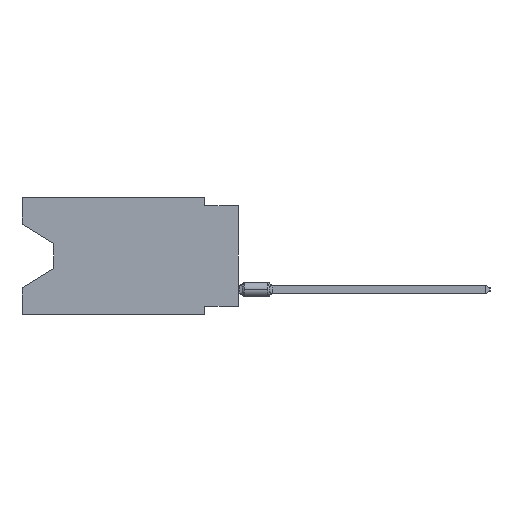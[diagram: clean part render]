
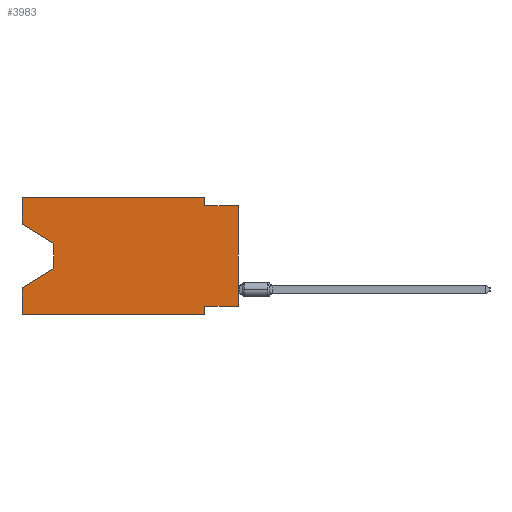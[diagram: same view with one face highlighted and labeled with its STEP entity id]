
A CAD part, left-side view. The second image highlights one B-rep face of the part: STEP entity #3983.
In plain terms, the highlighted planar face has unit normal (-1, 0, 0).
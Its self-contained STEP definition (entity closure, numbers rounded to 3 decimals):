
#249 = DIRECTION ( 'NONE',  ( 0., 0., 1. ) ) ;
#2544 = EDGE_CURVE ( 'NONE', #77701, #32352, #34237, .T. ) ;
#3983 = ADVANCED_FACE ( 'NONE', ( #42698 ), #12333, .F. ) ;
#5092 = DIRECTION ( 'NONE',  ( 0., 0., -1. ) ) ;
#7865 = VECTOR ( 'NONE', #76182, 1000. ) ;
#8477 = DIRECTION ( 'NONE',  ( 0., 1., 0. ) ) ;
#9603 = VECTOR ( 'NONE', #49959, 1000. ) ;
#9674 = CARTESIAN_POINT ( 'NONE',  ( 0., 0., -8.255 ) ) ;
#10720 = ORIENTED_EDGE ( 'NONE', *, *, #47616, .F. ) ;
#11368 = DIRECTION ( 'NONE',  ( 0., 0., 1. ) ) ;
#11590 = CARTESIAN_POINT ( 'NONE',  ( 0., 16.383, 0. ) ) ;
#12333 = PLANE ( 'NONE',  #65677 ) ;
#13125 = CARTESIAN_POINT ( 'NONE',  ( 0., 0., -0.635 ) ) ;
#13691 = VERTEX_POINT ( 'NONE', #33695 ) ;
#14118 = EDGE_LOOP ( 'NONE', ( #53825, #48049, #63645, #10720, #72800, #54632, #21055, #39411, #59504, #50692, #37069, #33156 ) ) ;
#15227 = DIRECTION ( 'NONE',  ( 0., -1., 0. ) ) ;
#15366 = VECTOR ( 'NONE', #54154, 1000. ) ;
#15761 = LINE ( 'NONE', #9674, #18253 ) ;
#17063 = VERTEX_POINT ( 'NONE', #44569 ) ;
#18253 = VECTOR ( 'NONE', #8477, 1000. ) ;
#20013 = VERTEX_POINT ( 'NONE', #76857 ) ;
#21055 = ORIENTED_EDGE ( 'NONE', *, *, #52044, .F. ) ;
#21905 = VERTEX_POINT ( 'NONE', #74834 ) ;
#25307 = LINE ( 'NONE', #79492, #9603 ) ;
#28143 = VERTEX_POINT ( 'NONE', #28400 ) ;
#28400 = CARTESIAN_POINT ( 'NONE',  ( 0., 2.54, -8.255 ) ) ;
#28641 = CARTESIAN_POINT ( 'NONE',  ( 0., 2.54, 0. ) ) ;
#30608 = LINE ( 'NONE', #11590, #71094 ) ;
#30962 = CARTESIAN_POINT ( 'NONE',  ( 0., 2.54, -0.635 ) ) ;
#31769 = CARTESIAN_POINT ( 'NONE',  ( 0., 2.54, 0. ) ) ;
#32124 = LINE ( 'NONE', #62843, #7865 ) ;
#32352 = VERTEX_POINT ( 'NONE', #72985 ) ;
#33156 = ORIENTED_EDGE ( 'NONE', *, *, #76078, .F. ) ;
#33184 = VECTOR ( 'NONE', #67475, 1000. ) ;
#33695 = CARTESIAN_POINT ( 'NONE',  ( 0., 0., -0.635 ) ) ;
#34237 = LINE ( 'NONE', #58502, #55093 ) ;
#35611 = EDGE_CURVE ( 'NONE', #21905, #17063, #32124, .T. ) ;
#36642 = LINE ( 'NONE', #31769, #58077 ) ;
#37069 = ORIENTED_EDGE ( 'NONE', *, *, #60213, .F. ) ;
#38857 = CARTESIAN_POINT ( 'NONE',  ( 0., 16.383, 0. ) ) ;
#39411 = ORIENTED_EDGE ( 'NONE', *, *, #66450, .T. ) ;
#39468 = VERTEX_POINT ( 'NONE', #38857 ) ;
#40224 = DIRECTION ( 'NONE',  ( 0., -1., 0. ) ) ;
#40738 = EDGE_CURVE ( 'NONE', #61234, #20013, #78411, .T. ) ;
#41652 = CARTESIAN_POINT ( 'NONE',  ( 0., 16.383, 0. ) ) ;
#41733 = CARTESIAN_POINT ( 'NONE',  ( 0., 0., 0. ) ) ;
#42698 = FACE_OUTER_BOUND ( 'NONE', #14118, .T. ) ;
#44569 = CARTESIAN_POINT ( 'NONE',  ( 0., 16.383, -6.852 ) ) ;
#45139 = EDGE_CURVE ( 'NONE', #20013, #21905, #25307, .T. ) ;
#46511 = VECTOR ( 'NONE', #62462, 1000. ) ;
#47616 = EDGE_CURVE ( 'NONE', #77701, #17063, #48108, .T. ) ;
#47877 = LINE ( 'NONE', #66467, #68755 ) ;
#48049 = ORIENTED_EDGE ( 'NONE', *, *, #45139, .T. ) ;
#48108 = LINE ( 'NONE', #41652, #33184 ) ;
#49320 = VERTEX_POINT ( 'NONE', #71123 ) ;
#49959 = DIRECTION ( 'NONE',  ( 0., 0., -1. ) ) ;
#50362 = EDGE_CURVE ( 'NONE', #28143, #32352, #63174, .T. ) ;
#50692 = ORIENTED_EDGE ( 'NONE', *, *, #67347, .F. ) ;
#51031 = CARTESIAN_POINT ( 'NONE',  ( 0., 2.54, -8.89 ) ) ;
#52044 = EDGE_CURVE ( 'NONE', #49320, #28143, #15761, .T. ) ;
#53682 = CARTESIAN_POINT ( 'NONE',  ( 0., 16.383, -8.89 ) ) ;
#53825 = ORIENTED_EDGE ( 'NONE', *, *, #40738, .T. ) ;
#54154 = DIRECTION ( 'NONE',  ( 0., -0.855, -0.519 ) ) ;
#54279 = CARTESIAN_POINT ( 'NONE',  ( 0., 16.383, -2.038 ) ) ;
#54430 = DIRECTION ( 'NONE',  ( 1., 0., 0. ) ) ;
#54632 = ORIENTED_EDGE ( 'NONE', *, *, #50362, .F. ) ;
#55093 = VECTOR ( 'NONE', #15227, 1000. ) ;
#55229 = CARTESIAN_POINT ( 'NONE',  ( 0., 16.383, 0. ) ) ;
#55234 = VECTOR ( 'NONE', #75303, 1000. ) ;
#58077 = VECTOR ( 'NONE', #68159, 1000. ) ;
#58502 = CARTESIAN_POINT ( 'NONE',  ( 0., 16.383, -8.89 ) ) ;
#59504 = ORIENTED_EDGE ( 'NONE', *, *, #70674, .F. ) ;
#60213 = EDGE_CURVE ( 'NONE', #39468, #77691, #47877, .T. ) ;
#60482 = LINE ( 'NONE', #13125, #46511 ) ;
#61234 = VERTEX_POINT ( 'NONE', #54279 ) ;
#62462 = DIRECTION ( 'NONE',  ( 0., -1., 0. ) ) ;
#62843 = CARTESIAN_POINT ( 'NONE',  ( 0., 13.97, -5.385 ) ) ;
#63174 = LINE ( 'NONE', #51031, #55234 ) ;
#63645 = ORIENTED_EDGE ( 'NONE', *, *, #35611, .T. ) ;
#65677 = AXIS2_PLACEMENT_3D ( 'NONE', #55229, #54430, #5092 ) ;
#66450 = EDGE_CURVE ( 'NONE', #49320, #13691, #66776, .T. ) ;
#66467 = CARTESIAN_POINT ( 'NONE',  ( 0., 16.383, 0. ) ) ;
#66776 = LINE ( 'NONE', #41733, #68287 ) ;
#67347 = EDGE_CURVE ( 'NONE', #77691, #71797, #36642, .T. ) ;
#67475 = DIRECTION ( 'NONE',  ( 0., 0., 1. ) ) ;
#68159 = DIRECTION ( 'NONE',  ( 0., 0., -1. ) ) ;
#68287 = VECTOR ( 'NONE', #11368, 1000. ) ;
#68755 = VECTOR ( 'NONE', #40224, 1000. ) ;
#70674 = EDGE_CURVE ( 'NONE', #71797, #13691, #60482, .T. ) ;
#71094 = VECTOR ( 'NONE', #249, 1000. ) ;
#71123 = CARTESIAN_POINT ( 'NONE',  ( 0., 0., -8.255 ) ) ;
#71563 = CARTESIAN_POINT ( 'NONE',  ( 0., 16.383, -2.038 ) ) ;
#71797 = VERTEX_POINT ( 'NONE', #30962 ) ;
#72800 = ORIENTED_EDGE ( 'NONE', *, *, #2544, .T. ) ;
#72985 = CARTESIAN_POINT ( 'NONE',  ( 0., 2.54, -8.89 ) ) ;
#74834 = CARTESIAN_POINT ( 'NONE',  ( 0., 13.97, -5.385 ) ) ;
#75303 = DIRECTION ( 'NONE',  ( 0., 0., -1. ) ) ;
#76078 = EDGE_CURVE ( 'NONE', #61234, #39468, #30608, .T. ) ;
#76182 = DIRECTION ( 'NONE',  ( 0., 0.855, -0.519 ) ) ;
#76857 = CARTESIAN_POINT ( 'NONE',  ( 0., 13.97, -3.505 ) ) ;
#77691 = VERTEX_POINT ( 'NONE', #28641 ) ;
#77701 = VERTEX_POINT ( 'NONE', #53682 ) ;
#78411 = LINE ( 'NONE', #71563, #15366 ) ;
#79492 = CARTESIAN_POINT ( 'NONE',  ( 0., 13.97, -3.505 ) ) ;
